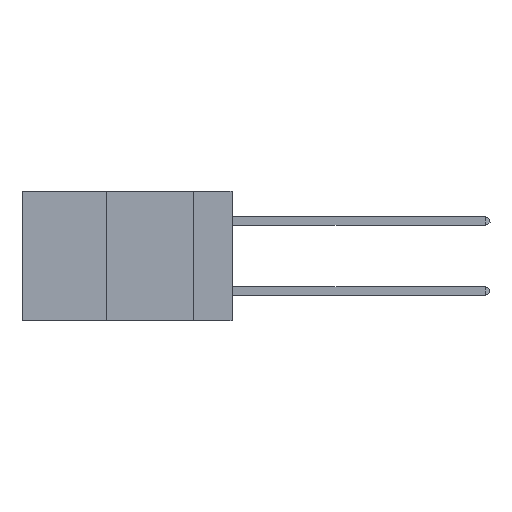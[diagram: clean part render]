
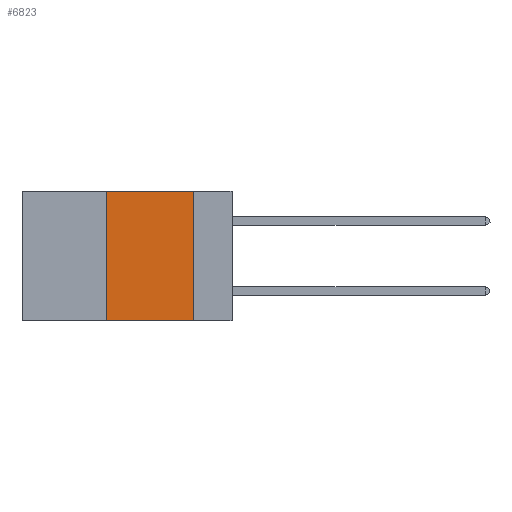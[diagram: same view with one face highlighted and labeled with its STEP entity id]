
A CAD part, left-side view. The second image highlights one B-rep face of the part: STEP entity #6823.
In plain terms, the highlighted planar face has unit normal (-1, 0, 0).
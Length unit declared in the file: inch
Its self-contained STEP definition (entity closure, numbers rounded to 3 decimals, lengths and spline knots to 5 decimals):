
#341 = DIRECTION ( 'NONE',  ( 0., 0., -1. ) ) ;
#792 = LINE ( 'NONE', #5661, #11737 ) ;
#999 = LINE ( 'NONE', #2619, #3128 ) ;
#2052 = ORIENTED_EDGE ( 'NONE', *, *, #7094, .F. ) ;
#2619 = CARTESIAN_POINT ( 'NONE',  ( 0., 0.6, 0. ) ) ;
#2745 = CARTESIAN_POINT ( 'NONE',  ( 0., 0.36, 0. ) ) ;
#2974 = DIRECTION ( 'NONE',  ( 0., -1., 0. ) ) ;
#3128 = VECTOR ( 'NONE', #18165, 39.37008 ) ;
#3882 = VECTOR ( 'NONE', #2974, 39.37008 ) ;
#4586 = PLANE ( 'NONE',  #24897 ) ;
#4854 = VERTEX_POINT ( 'NONE', #15899 ) ;
#5224 = ORIENTED_EDGE ( 'NONE', *, *, #12106, .F. ) ;
#5661 = CARTESIAN_POINT ( 'NONE',  ( 0., 0.36, 0. ) ) ;
#6067 = VERTEX_POINT ( 'NONE', #2745 ) ;
#6823 = ADVANCED_FACE ( 'NONE', ( #18612 ), #4586, .F. ) ;
#7094 = EDGE_CURVE ( 'NONE', #6067, #4854, #999, .T. ) ;
#7345 = LINE ( 'NONE', #10041, #14625 ) ;
#8357 = CARTESIAN_POINT ( 'NONE',  ( 0., 0.11, -0.37 ) ) ;
#8795 = LINE ( 'NONE', #14628, #3882 ) ;
#10041 = CARTESIAN_POINT ( 'NONE',  ( 0., 0.11, 0. ) ) ;
#11575 = VERTEX_POINT ( 'NONE', #20042 ) ;
#11737 = VECTOR ( 'NONE', #17274, 39.37008 ) ;
#12106 = EDGE_CURVE ( 'NONE', #4854, #15863, #7345, .T. ) ;
#12347 = CARTESIAN_POINT ( 'NONE',  ( 0., 0.6, 0. ) ) ;
#14625 = VECTOR ( 'NONE', #341, 39.37008 ) ;
#14628 = CARTESIAN_POINT ( 'NONE',  ( 0., 0.6, -0.37 ) ) ;
#15863 = VERTEX_POINT ( 'NONE', #8357 ) ;
#15899 = CARTESIAN_POINT ( 'NONE',  ( 0., 0.11, 0. ) ) ;
#16452 = EDGE_LOOP ( 'NONE', ( #5224, #2052, #22724, #21276 ) ) ;
#17274 = DIRECTION ( 'NONE',  ( 0., 0., 1. ) ) ;
#18165 = DIRECTION ( 'NONE',  ( 0., -1., 0. ) ) ;
#18612 = FACE_OUTER_BOUND ( 'NONE', #16452, .T. ) ;
#20042 = CARTESIAN_POINT ( 'NONE',  ( 0., 0.36, -0.37 ) ) ;
#20166 = DIRECTION ( 'NONE',  ( 0., 0., -1. ) ) ;
#21276 = ORIENTED_EDGE ( 'NONE', *, *, #24892, .T. ) ;
#21823 = EDGE_CURVE ( 'NONE', #11575, #6067, #792, .T. ) ;
#22724 = ORIENTED_EDGE ( 'NONE', *, *, #21823, .F. ) ;
#23753 = DIRECTION ( 'NONE',  ( 1., 0., 0. ) ) ;
#24892 = EDGE_CURVE ( 'NONE', #11575, #15863, #8795, .T. ) ;
#24897 = AXIS2_PLACEMENT_3D ( 'NONE', #12347, #23753, #20166 ) ;
